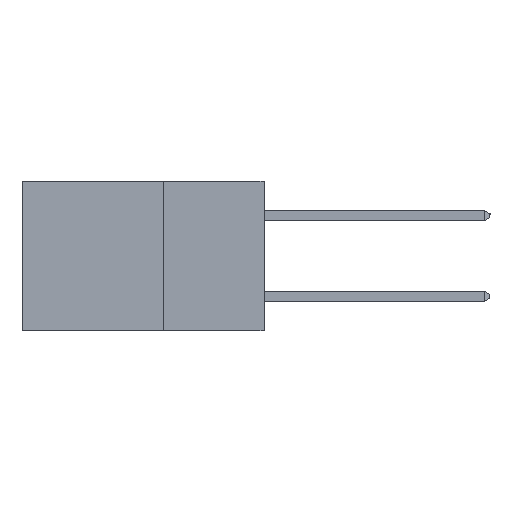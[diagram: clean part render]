
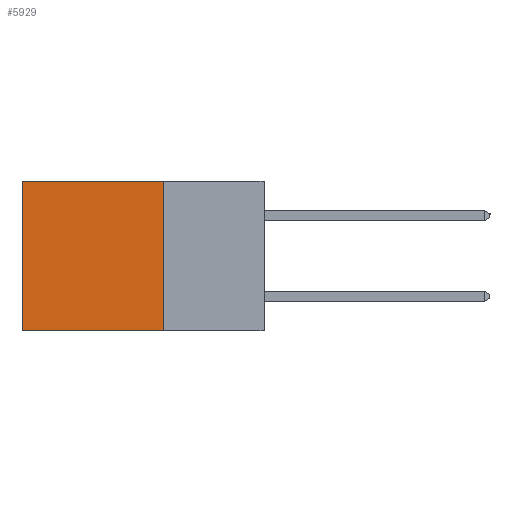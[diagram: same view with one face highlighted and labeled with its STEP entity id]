
A CAD part, left-side view. The second image highlights one B-rep face of the part: STEP entity #5929.
In plain terms, the highlighted planar face has unit normal (-1, 0, 0).
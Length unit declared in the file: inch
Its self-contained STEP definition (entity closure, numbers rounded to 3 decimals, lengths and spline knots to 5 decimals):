
#485 = CARTESIAN_POINT ( 'NONE',  ( 0.298, 0.25, 0. ) ) ;
#926 = DIRECTION ( 'NONE',  ( 0., 0., -1. ) ) ;
#1077 = CARTESIAN_POINT ( 'NONE',  ( 0.298, 0.6, -0.37 ) ) ;
#1216 = ORIENTED_EDGE ( 'NONE', *, *, #10698, .F. ) ;
#1297 = DIRECTION ( 'NONE',  ( 0., 0., -1. ) ) ;
#1517 = CARTESIAN_POINT ( 'NONE',  ( 0.298, 0.6, 0. ) ) ;
#1947 = CARTESIAN_POINT ( 'NONE',  ( 0.298, 0.25, 0. ) ) ;
#2293 = EDGE_LOOP ( 'NONE', ( #8120, #4161, #1216, #14295 ) ) ;
#3741 = VECTOR ( 'NONE', #12776, 39.37008 ) ;
#3868 = CARTESIAN_POINT ( 'NONE',  ( 0.298, 0.25, 0. ) ) ;
#4131 = LINE ( 'NONE', #485, #3741 ) ;
#4161 = ORIENTED_EDGE ( 'NONE', *, *, #6816, .F. ) ;
#4830 = LINE ( 'NONE', #3868, #9160 ) ;
#5774 = VERTEX_POINT ( 'NONE', #11621 ) ;
#5775 = AXIS2_PLACEMENT_3D ( 'NONE', #1947, #10312, #926 ) ;
#5929 = ADVANCED_FACE ( 'NONE', ( #11389 ), #7862, .F. ) ;
#6816 = EDGE_CURVE ( 'NONE', #5774, #15271, #11763, .T. ) ;
#7413 = CARTESIAN_POINT ( 'NONE',  ( 0.298, 0.6, 0. ) ) ;
#7862 = PLANE ( 'NONE',  #5775 ) ;
#8120 = ORIENTED_EDGE ( 'NONE', *, *, #8511, .T. ) ;
#8511 = EDGE_CURVE ( 'NONE', #11950, #15271, #9170, .T. ) ;
#9102 = VERTEX_POINT ( 'NONE', #15733 ) ;
#9160 = VECTOR ( 'NONE', #11170, 39.37008 ) ;
#9170 = LINE ( 'NONE', #7413, #15292 ) ;
#10312 = DIRECTION ( 'NONE',  ( 1., 0., 0. ) ) ;
#10698 = EDGE_CURVE ( 'NONE', #9102, #5774, #4131, .T. ) ;
#10763 = CARTESIAN_POINT ( 'NONE',  ( 0.298, 0.25, -0.37 ) ) ;
#10786 = DIRECTION ( 'NONE',  ( 0., 1., 0. ) ) ;
#11170 = DIRECTION ( 'NONE',  ( 0., 1., 0. ) ) ;
#11357 = VECTOR ( 'NONE', #10786, 39.37008 ) ;
#11389 = FACE_OUTER_BOUND ( 'NONE', #2293, .T. ) ;
#11621 = CARTESIAN_POINT ( 'NONE',  ( 0.298, 0.25, -0.37 ) ) ;
#11763 = LINE ( 'NONE', #10763, #11357 ) ;
#11950 = VERTEX_POINT ( 'NONE', #1517 ) ;
#12776 = DIRECTION ( 'NONE',  ( 0., 0., -1. ) ) ;
#13282 = EDGE_CURVE ( 'NONE', #9102, #11950, #4830, .T. ) ;
#14295 = ORIENTED_EDGE ( 'NONE', *, *, #13282, .T. ) ;
#15271 = VERTEX_POINT ( 'NONE', #1077 ) ;
#15292 = VECTOR ( 'NONE', #1297, 39.37008 ) ;
#15733 = CARTESIAN_POINT ( 'NONE',  ( 0.298, 0.25, 0. ) ) ;
